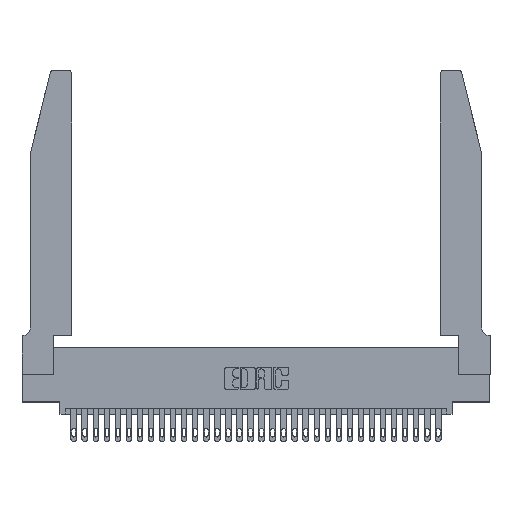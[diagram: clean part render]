
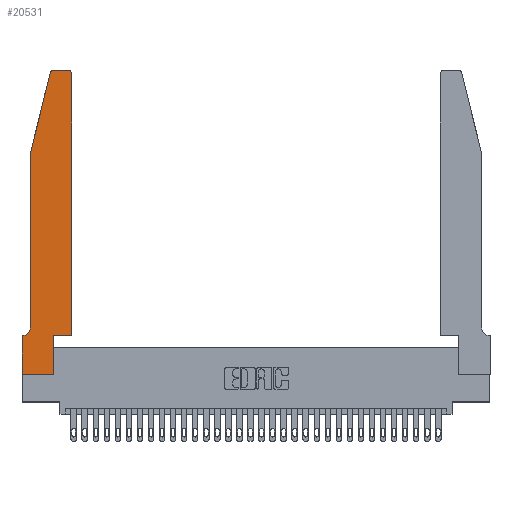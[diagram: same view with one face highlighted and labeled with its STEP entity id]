
A CAD part, top view. The second image highlights one B-rep face of the part: STEP entity #20531.
In plain terms, the highlighted planar face has unit normal (0, 0, 1).
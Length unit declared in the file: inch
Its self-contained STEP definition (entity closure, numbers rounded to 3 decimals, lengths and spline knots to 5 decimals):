
#581 = AXIS2_PLACEMENT_3D ( 'NONE', #8186, #3574, #10919 ) ;
#748 = CARTESIAN_POINT ( 'NONE',  ( 0.0755, 0.42, 0.37 ) ) ;
#842 = CARTESIAN_POINT ( 'NONE',  ( 0., 0.35, 0.37 ) ) ;
#913 = DIRECTION ( 'NONE',  ( 0., 0., 1. ) ) ;
#993 = EDGE_CURVE ( 'NONE', #10211, #30217, #2769, .T. ) ;
#1116 = DIRECTION ( 'NONE',  ( 1., 0., 0. ) ) ;
#1158 = EDGE_CURVE ( 'NONE', #30217, #17672, #18089, .T. ) ;
#1429 = DIRECTION ( 'NONE',  ( 0., 0., 1. ) ) ;
#1472 = DIRECTION ( 'NONE',  ( -1., 0., 0. ) ) ;
#1544 = FACE_OUTER_BOUND ( 'NONE', #2363, .T. ) ;
#1823 = CIRCLE ( 'NONE', #4381, 0.03 ) ;
#1834 = CARTESIAN_POINT ( 'NONE',  ( 0., 0., 0.37 ) ) ;
#2263 = ORIENTED_EDGE ( 'NONE', *, *, #21476, .T. ) ;
#2363 = EDGE_LOOP ( 'NONE', ( #28621, #21394, #24220, #24087, #31043, #2263, #22779, #4668, #28067, #9359, #23162, #13455 ) ) ;
#2769 = LINE ( 'NONE', #1834, #8686 ) ;
#2835 = CARTESIAN_POINT ( 'NONE',  ( 0.25487, 2.72718, 0.37 ) ) ;
#3485 = DIRECTION ( 'NONE',  ( 1., 0., 0. ) ) ;
#3574 = DIRECTION ( 'NONE',  ( 0., 0., -1. ) ) ;
#4084 = DIRECTION ( 'NONE',  ( 0., -1., 0. ) ) ;
#4112 = EDGE_CURVE ( 'NONE', #5878, #16964, #20103, .T. ) ;
#4309 = EDGE_CURVE ( 'NONE', #5830, #19943, #8292, .T. ) ;
#4381 = AXIS2_PLACEMENT_3D ( 'NONE', #16467, #913, #3485 ) ;
#4634 = VERTEX_POINT ( 'NONE', #748 ) ;
#4668 = ORIENTED_EDGE ( 'NONE', *, *, #1158, .T. ) ;
#4795 = VECTOR ( 'NONE', #1472, 39.37008 ) ;
#5742 = EDGE_CURVE ( 'NONE', #29257, #15029, #30984, .T. ) ;
#5830 = VERTEX_POINT ( 'NONE', #19096 ) ;
#5878 = VERTEX_POINT ( 'NONE', #29955 ) ;
#5913 = DIRECTION ( 'NONE',  ( -1., 0., 0. ) ) ;
#7158 = VECTOR ( 'NONE', #19622, 39.37008 ) ;
#7911 = LINE ( 'NONE', #15912, #19734 ) ;
#8186 = CARTESIAN_POINT ( 'NONE',  ( 0.0055, 0.42, 0.37 ) ) ;
#8246 = EDGE_CURVE ( 'NONE', #25856, #5830, #31507, .T. ) ;
#8292 = LINE ( 'NONE', #29751, #27544 ) ;
#8438 = CARTESIAN_POINT ( 'NONE',  ( 0.0755, 2., 0.37 ) ) ;
#8686 = VECTOR ( 'NONE', #14622, 39.37008 ) ;
#8809 = EDGE_CURVE ( 'NONE', #16964, #29257, #15442, .T. ) ;
#9324 = LINE ( 'NONE', #15944, #10467 ) ;
#9359 = ORIENTED_EDGE ( 'NONE', *, *, #8246, .T. ) ;
#9764 = CARTESIAN_POINT ( 'NONE',  ( 0.2865, 0.35, 0.37 ) ) ;
#10211 = VERTEX_POINT ( 'NONE', #842 ) ;
#10288 = EDGE_CURVE ( 'NONE', #17672, #25856, #10555, .T. ) ;
#10467 = VECTOR ( 'NONE', #4084, 39.37008 ) ;
#10555 = LINE ( 'NONE', #22201, #14542 ) ;
#10919 = DIRECTION ( 'NONE',  ( -1., 0., 0. ) ) ;
#11360 = DIRECTION ( 'NONE',  ( 1., 0., 0. ) ) ;
#11448 = CIRCLE ( 'NONE', #581, 0.07 ) ;
#12388 = EDGE_CURVE ( 'NONE', #15029, #4634, #9324, .T. ) ;
#13455 = ORIENTED_EDGE ( 'NONE', *, *, #15693, .T. ) ;
#14542 = VECTOR ( 'NONE', #27625, 39.37008 ) ;
#14622 = DIRECTION ( 'NONE',  ( 0., -1., 0. ) ) ;
#15029 = VERTEX_POINT ( 'NONE', #8438 ) ;
#15442 = CIRCLE ( 'NONE', #17639, 0.03 ) ;
#15693 = EDGE_CURVE ( 'NONE', #19943, #5878, #1823, .T. ) ;
#15912 = CARTESIAN_POINT ( 'NONE',  ( 0.0755, 0.35, 0.37 ) ) ;
#15944 = CARTESIAN_POINT ( 'NONE',  ( 0.0755, 2., 0.37 ) ) ;
#16455 = CARTESIAN_POINT ( 'NONE',  ( 0.2605, 2.75, 0.37 ) ) ;
#16467 = CARTESIAN_POINT ( 'NONE',  ( 0.4205, 2.72, 0.37 ) ) ;
#16527 = CARTESIAN_POINT ( 'NONE',  ( 0., 0.35, 0.37 ) ) ;
#16543 = VECTOR ( 'NONE', #1116, 39.37008 ) ;
#16964 = VERTEX_POINT ( 'NONE', #21669 ) ;
#17225 = CARTESIAN_POINT ( 'NONE',  ( 0.2865, 0., 0.37 ) ) ;
#17639 = AXIS2_PLACEMENT_3D ( 'NONE', #24318, #29065, #26638 ) ;
#17672 = VERTEX_POINT ( 'NONE', #17225 ) ;
#18089 = LINE ( 'NONE', #23637, #16543 ) ;
#19096 = CARTESIAN_POINT ( 'NONE',  ( 0.4505, 0.35, 0.37 ) ) ;
#19210 = CARTESIAN_POINT ( 'NONE',  ( 0.0755, 2., 0.37 ) ) ;
#19233 = VECTOR ( 'NONE', #19310, 39.37008 ) ;
#19310 = DIRECTION ( 'NONE',  ( -0.239, -0.971, 0. ) ) ;
#19622 = DIRECTION ( 'NONE',  ( 1., 0., 0. ) ) ;
#19734 = VECTOR ( 'NONE', #5913, 39.37008 ) ;
#19943 = VERTEX_POINT ( 'NONE', #25862 ) ;
#19968 = EDGE_CURVE ( 'NONE', #4634, #21932, #11448, .T. ) ;
#20103 = LINE ( 'NONE', #16455, #4795 ) ;
#20531 = ADVANCED_FACE ( 'NONE', ( #1544 ), #24079, .T. ) ;
#21394 = ORIENTED_EDGE ( 'NONE', *, *, #8809, .T. ) ;
#21476 = EDGE_CURVE ( 'NONE', #21932, #10211, #7911, .T. ) ;
#21604 = CARTESIAN_POINT ( 'NONE',  ( 0., 0., 0.37 ) ) ;
#21669 = CARTESIAN_POINT ( 'NONE',  ( 0.284, 2.75, 0.37 ) ) ;
#21932 = VERTEX_POINT ( 'NONE', #23082 ) ;
#22201 = CARTESIAN_POINT ( 'NONE',  ( 0.2865, 0.35, 0.37 ) ) ;
#22779 = ORIENTED_EDGE ( 'NONE', *, *, #993, .T. ) ;
#23082 = CARTESIAN_POINT ( 'NONE',  ( 0.0055, 0.35, 0.37 ) ) ;
#23162 = ORIENTED_EDGE ( 'NONE', *, *, #4309, .T. ) ;
#23637 = CARTESIAN_POINT ( 'NONE',  ( 0., 0., 0.37 ) ) ;
#24079 = PLANE ( 'NONE',  #25096 ) ;
#24087 = ORIENTED_EDGE ( 'NONE', *, *, #12388, .T. ) ;
#24220 = ORIENTED_EDGE ( 'NONE', *, *, #5742, .T. ) ;
#24318 = CARTESIAN_POINT ( 'NONE',  ( 0.284, 2.72, 0.37 ) ) ;
#25096 = AXIS2_PLACEMENT_3D ( 'NONE', #16527, #1429, #11360 ) ;
#25856 = VERTEX_POINT ( 'NONE', #9764 ) ;
#25862 = CARTESIAN_POINT ( 'NONE',  ( 0.4505, 2.72, 0.37 ) ) ;
#26638 = DIRECTION ( 'NONE',  ( 1., 0., 0. ) ) ;
#27001 = DIRECTION ( 'NONE',  ( 0., 1., 0. ) ) ;
#27062 = CARTESIAN_POINT ( 'NONE',  ( 0.4505, 0.35, 0.37 ) ) ;
#27544 = VECTOR ( 'NONE', #27001, 39.37008 ) ;
#27625 = DIRECTION ( 'NONE',  ( 0., 1., 0. ) ) ;
#28067 = ORIENTED_EDGE ( 'NONE', *, *, #10288, .T. ) ;
#28621 = ORIENTED_EDGE ( 'NONE', *, *, #4112, .T. ) ;
#29065 = DIRECTION ( 'NONE',  ( 0., 0., 1. ) ) ;
#29257 = VERTEX_POINT ( 'NONE', #2835 ) ;
#29751 = CARTESIAN_POINT ( 'NONE',  ( 0.4505, 0.35, 0.37 ) ) ;
#29955 = CARTESIAN_POINT ( 'NONE',  ( 0.4205, 2.75, 0.37 ) ) ;
#30217 = VERTEX_POINT ( 'NONE', #21604 ) ;
#30984 = LINE ( 'NONE', #19210, #19233 ) ;
#31043 = ORIENTED_EDGE ( 'NONE', *, *, #19968, .T. ) ;
#31507 = LINE ( 'NONE', #27062, #7158 ) ;
